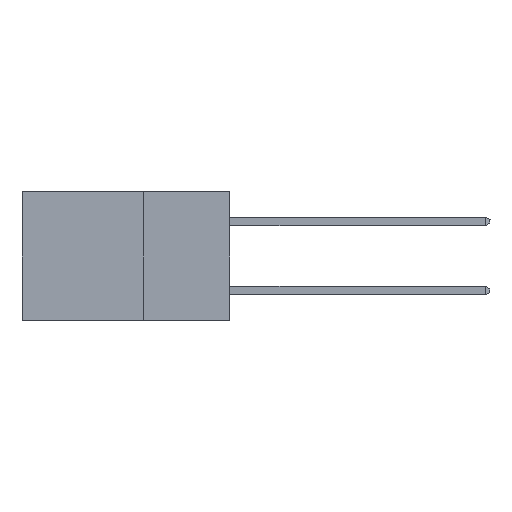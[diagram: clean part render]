
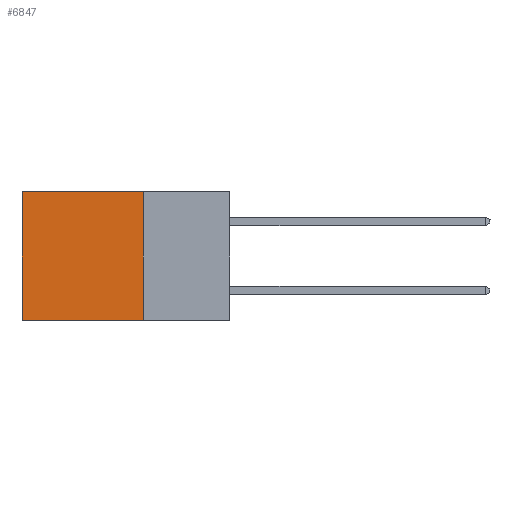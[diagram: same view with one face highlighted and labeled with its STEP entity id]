
A CAD part, left-side view. The second image highlights one B-rep face of the part: STEP entity #6847.
In plain terms, the highlighted planar face has unit normal (-1, 0, 0).
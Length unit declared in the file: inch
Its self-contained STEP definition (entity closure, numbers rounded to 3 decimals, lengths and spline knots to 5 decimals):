
#182 = CARTESIAN_POINT ( 'NONE',  ( 0.2615, 0.25, -0.37 ) ) ;
#375 = LINE ( 'NONE', #11485, #6047 ) ;
#410 = CARTESIAN_POINT ( 'NONE',  ( 0.2615, 0.25, -0.37 ) ) ;
#523 = LINE ( 'NONE', #9101, #3956 ) ;
#1236 = EDGE_CURVE ( 'NONE', #10537, #1554, #6266, .T. ) ;
#1554 = VERTEX_POINT ( 'NONE', #12124 ) ;
#2815 = EDGE_CURVE ( 'NONE', #9142, #1554, #523, .T. ) ;
#2977 = ORIENTED_EDGE ( 'NONE', *, *, #1236, .T. ) ;
#3476 = VERTEX_POINT ( 'NONE', #16016 ) ;
#3956 = VECTOR ( 'NONE', #6537, 39.37008 ) ;
#3988 = PLANE ( 'NONE',  #8896 ) ;
#5064 = FACE_OUTER_BOUND ( 'NONE', #10812, .T. ) ;
#5218 = DIRECTION ( 'NONE',  ( 0., 0., -1. ) ) ;
#5612 = LINE ( 'NONE', #410, #14180 ) ;
#6047 = VECTOR ( 'NONE', #8868, 39.37008 ) ;
#6266 = LINE ( 'NONE', #14913, #6741 ) ;
#6498 = DIRECTION ( 'NONE',  ( 1., 0., 0. ) ) ;
#6537 = DIRECTION ( 'NONE',  ( 0., 1., 0. ) ) ;
#6741 = VECTOR ( 'NONE', #11195, 39.37008 ) ;
#6847 = ADVANCED_FACE ( 'NONE', ( #5064 ), #3988, .F. ) ;
#7084 = ORIENTED_EDGE ( 'NONE', *, *, #2815, .F. ) ;
#8868 = DIRECTION ( 'NONE',  ( 0., 1., 0. ) ) ;
#8896 = AXIS2_PLACEMENT_3D ( 'NONE', #182, #6498, #5218 ) ;
#9101 = CARTESIAN_POINT ( 'NONE',  ( 0.2615, 0.25, -0.37 ) ) ;
#9142 = VERTEX_POINT ( 'NONE', #9346 ) ;
#9346 = CARTESIAN_POINT ( 'NONE',  ( 0.2615, 0.25, -0.37 ) ) ;
#10143 = ORIENTED_EDGE ( 'NONE', *, *, #15397, .T. ) ;
#10313 = DIRECTION ( 'NONE',  ( 0., 0., -1. ) ) ;
#10537 = VERTEX_POINT ( 'NONE', #10576 ) ;
#10576 = CARTESIAN_POINT ( 'NONE',  ( 0.2615, 0.6, 0. ) ) ;
#10812 = EDGE_LOOP ( 'NONE', ( #2977, #7084, #15021, #10143 ) ) ;
#11195 = DIRECTION ( 'NONE',  ( 0., 0., -1. ) ) ;
#11461 = EDGE_CURVE ( 'NONE', #3476, #9142, #5612, .T. ) ;
#11485 = CARTESIAN_POINT ( 'NONE',  ( 0.2615, 0.25, 0. ) ) ;
#12124 = CARTESIAN_POINT ( 'NONE',  ( 0.2615, 0.6, -0.37 ) ) ;
#14180 = VECTOR ( 'NONE', #10313, 39.37008 ) ;
#14913 = CARTESIAN_POINT ( 'NONE',  ( 0.2615, 0.6, -0.37 ) ) ;
#15021 = ORIENTED_EDGE ( 'NONE', *, *, #11461, .F. ) ;
#15397 = EDGE_CURVE ( 'NONE', #3476, #10537, #375, .T. ) ;
#16016 = CARTESIAN_POINT ( 'NONE',  ( 0.2615, 0.25, 0. ) ) ;
